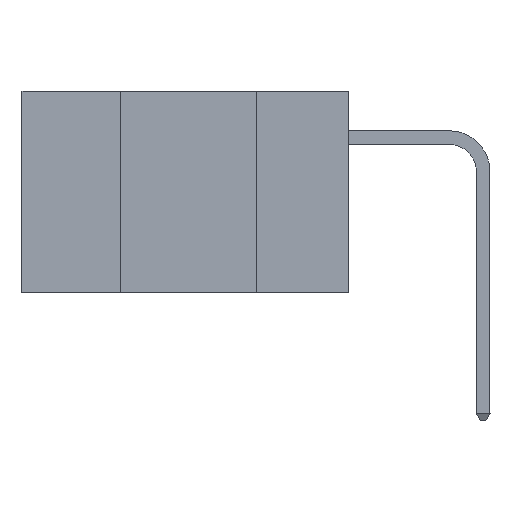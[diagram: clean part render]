
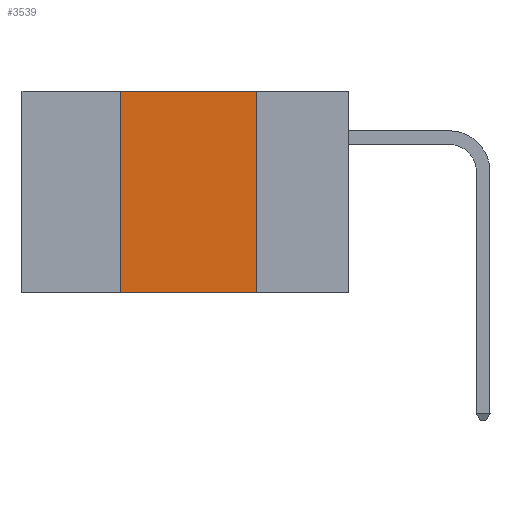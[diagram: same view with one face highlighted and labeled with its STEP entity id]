
A CAD part, left-side view. The second image highlights one B-rep face of the part: STEP entity #3539.
In plain terms, the highlighted planar face has unit normal (-1, 0, 0).
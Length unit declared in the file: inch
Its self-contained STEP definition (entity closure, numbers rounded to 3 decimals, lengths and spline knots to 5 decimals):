
#351 = LINE ( 'NONE', #2107, #16820 ) ;
#455 = CARTESIAN_POINT ( 'NONE',  ( 0., 0.17, 0. ) ) ;
#692 = AXIS2_PLACEMENT_3D ( 'NONE', #12355, #10787, #17103 ) ;
#2107 = CARTESIAN_POINT ( 'NONE',  ( 0., 0.6, -0.37 ) ) ;
#3539 = ADVANCED_FACE ( 'NONE', ( #7554 ), #13896, .F. ) ;
#4586 = CARTESIAN_POINT ( 'NONE',  ( 0., 0.17, 0. ) ) ;
#5579 = EDGE_CURVE ( 'NONE', #17235, #17756, #8008, .T. ) ;
#6333 = DIRECTION ( 'NONE',  ( 0., -1., 0. ) ) ;
#6641 = ORIENTED_EDGE ( 'NONE', *, *, #13626, .F. ) ;
#7394 = DIRECTION ( 'NONE',  ( 0., 0., -1. ) ) ;
#7417 = DIRECTION ( 'NONE',  ( 0., 0., 1. ) ) ;
#7554 = FACE_OUTER_BOUND ( 'NONE', #10928, .T. ) ;
#8008 = LINE ( 'NONE', #19991, #14548 ) ;
#8432 = DIRECTION ( 'NONE',  ( 0., -1., 0. ) ) ;
#8797 = VERTEX_POINT ( 'NONE', #13768 ) ;
#9914 = CARTESIAN_POINT ( 'NONE',  ( 0., 0.42, 0. ) ) ;
#10787 = DIRECTION ( 'NONE',  ( 1., 0., 0. ) ) ;
#10928 = EDGE_LOOP ( 'NONE', ( #13805, #6641, #20161, #18318 ) ) ;
#12355 = CARTESIAN_POINT ( 'NONE',  ( 0., 0.6, 0. ) ) ;
#13626 = EDGE_CURVE ( 'NONE', #17756, #18162, #14217, .T. ) ;
#13768 = CARTESIAN_POINT ( 'NONE',  ( 0., 0.17, -0.37 ) ) ;
#13805 = ORIENTED_EDGE ( 'NONE', *, *, #16668, .F. ) ;
#13896 = PLANE ( 'NONE',  #692 ) ;
#14217 = LINE ( 'NONE', #17230, #14368 ) ;
#14368 = VECTOR ( 'NONE', #6333, 39.37008 ) ;
#14548 = VECTOR ( 'NONE', #7417, 39.37008 ) ;
#16668 = EDGE_CURVE ( 'NONE', #18162, #8797, #17249, .T. ) ;
#16820 = VECTOR ( 'NONE', #8432, 39.37008 ) ;
#17096 = VECTOR ( 'NONE', #7394, 39.37008 ) ;
#17103 = DIRECTION ( 'NONE',  ( 0., 0., -1. ) ) ;
#17230 = CARTESIAN_POINT ( 'NONE',  ( 0., 0.6, 0. ) ) ;
#17235 = VERTEX_POINT ( 'NONE', #18754 ) ;
#17249 = LINE ( 'NONE', #4586, #17096 ) ;
#17756 = VERTEX_POINT ( 'NONE', #9914 ) ;
#18162 = VERTEX_POINT ( 'NONE', #455 ) ;
#18318 = ORIENTED_EDGE ( 'NONE', *, *, #19981, .T. ) ;
#18754 = CARTESIAN_POINT ( 'NONE',  ( 0., 0.42, -0.37 ) ) ;
#19981 = EDGE_CURVE ( 'NONE', #17235, #8797, #351, .T. ) ;
#19991 = CARTESIAN_POINT ( 'NONE',  ( 0., 0.42, 0. ) ) ;
#20161 = ORIENTED_EDGE ( 'NONE', *, *, #5579, .F. ) ;
